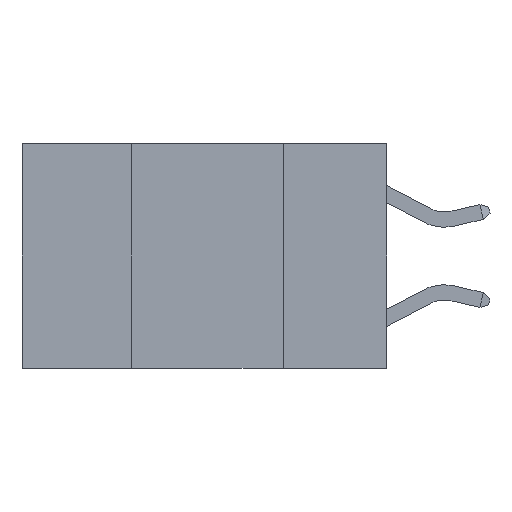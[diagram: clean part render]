
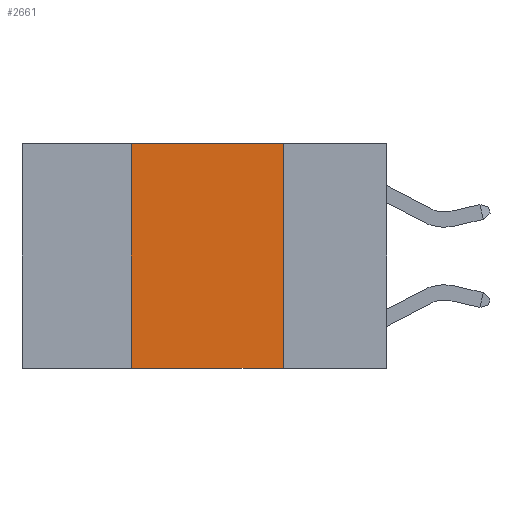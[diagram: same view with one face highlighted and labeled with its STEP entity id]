
A CAD part, left-side view. The second image highlights one B-rep face of the part: STEP entity #2661.
In plain terms, the highlighted planar face has unit normal (-1, 0, 0).
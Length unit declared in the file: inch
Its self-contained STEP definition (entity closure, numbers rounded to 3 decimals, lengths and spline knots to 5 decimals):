
#1173 = LINE ( 'NONE', #9787, #11624 ) ;
#1195 = AXIS2_PLACEMENT_3D ( 'NONE', #7441, #10501, #4450 ) ;
#1414 = VERTEX_POINT ( 'NONE', #6336 ) ;
#1619 = CARTESIAN_POINT ( 'NONE',  ( 0., 0.42, 0. ) ) ;
#2218 = CARTESIAN_POINT ( 'NONE',  ( 0., 0.17, 0. ) ) ;
#2275 = CARTESIAN_POINT ( 'NONE',  ( 0., 0.6, -0.37 ) ) ;
#2661 = ADVANCED_FACE ( 'NONE', ( #12442 ), #3406, .F. ) ;
#3249 = DIRECTION ( 'NONE',  ( 0., 0., -1. ) ) ;
#3406 = PLANE ( 'NONE',  #1195 ) ;
#3879 = CARTESIAN_POINT ( 'NONE',  ( 0., 0.42, -0.37 ) ) ;
#3895 = VECTOR ( 'NONE', #12103, 39.37008 ) ;
#4450 = DIRECTION ( 'NONE',  ( 0., 0., -1. ) ) ;
#4749 = VECTOR ( 'NONE', #3249, 39.37008 ) ;
#4884 = LINE ( 'NONE', #11100, #3895 ) ;
#5072 = LINE ( 'NONE', #2218, #4749 ) ;
#5680 = ORIENTED_EDGE ( 'NONE', *, *, #8584, .F. ) ;
#6302 = EDGE_CURVE ( 'NONE', #7976, #1414, #5072, .T. ) ;
#6336 = CARTESIAN_POINT ( 'NONE',  ( 0., 0.17, -0.37 ) ) ;
#6406 = DIRECTION ( 'NONE',  ( 0., -1., 0. ) ) ;
#7180 = EDGE_CURVE ( 'NONE', #9935, #1414, #7266, .T. ) ;
#7266 = LINE ( 'NONE', #2275, #9604 ) ;
#7441 = CARTESIAN_POINT ( 'NONE',  ( 0., 0.6, 0. ) ) ;
#7976 = VERTEX_POINT ( 'NONE', #8826 ) ;
#8124 = EDGE_CURVE ( 'NONE', #12681, #7976, #4884, .T. ) ;
#8584 = EDGE_CURVE ( 'NONE', #9935, #12681, #1173, .T. ) ;
#8826 = CARTESIAN_POINT ( 'NONE',  ( 0., 0.17, 0. ) ) ;
#9093 = ORIENTED_EDGE ( 'NONE', *, *, #8124, .F. ) ;
#9604 = VECTOR ( 'NONE', #6406, 39.37008 ) ;
#9694 = ORIENTED_EDGE ( 'NONE', *, *, #6302, .F. ) ;
#9787 = CARTESIAN_POINT ( 'NONE',  ( 0., 0.42, 0. ) ) ;
#9935 = VERTEX_POINT ( 'NONE', #3879 ) ;
#10501 = DIRECTION ( 'NONE',  ( 1., 0., 0. ) ) ;
#10540 = EDGE_LOOP ( 'NONE', ( #9694, #9093, #5680, #12784 ) ) ;
#11100 = CARTESIAN_POINT ( 'NONE',  ( 0., 0.6, 0. ) ) ;
#11624 = VECTOR ( 'NONE', #12787, 39.37008 ) ;
#12103 = DIRECTION ( 'NONE',  ( 0., -1., 0. ) ) ;
#12442 = FACE_OUTER_BOUND ( 'NONE', #10540, .T. ) ;
#12681 = VERTEX_POINT ( 'NONE', #1619 ) ;
#12784 = ORIENTED_EDGE ( 'NONE', *, *, #7180, .T. ) ;
#12787 = DIRECTION ( 'NONE',  ( 0., 0., 1. ) ) ;
